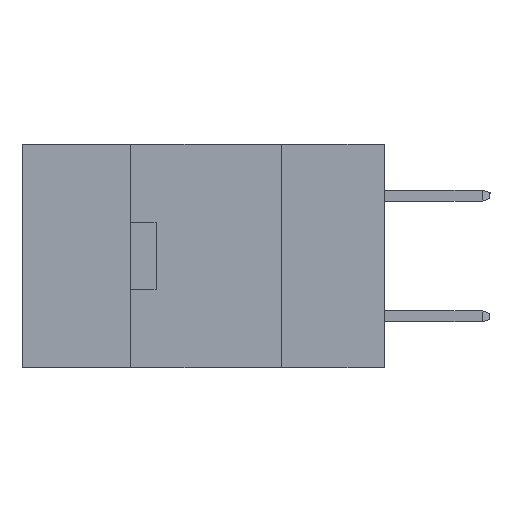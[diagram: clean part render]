
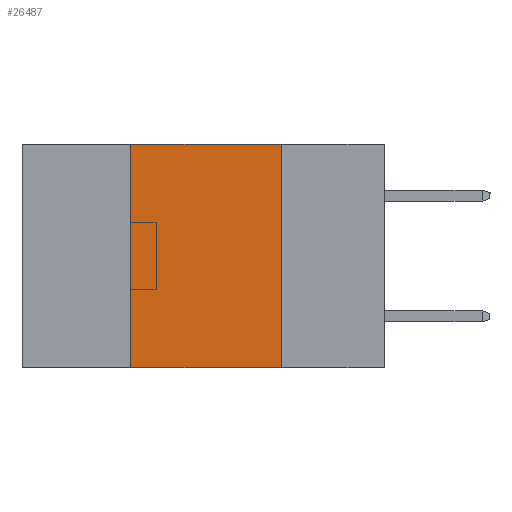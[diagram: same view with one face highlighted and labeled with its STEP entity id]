
A CAD part, left-side view. The second image highlights one B-rep face of the part: STEP entity #26487.
In plain terms, the highlighted planar face has unit normal (-1, 0, 0).
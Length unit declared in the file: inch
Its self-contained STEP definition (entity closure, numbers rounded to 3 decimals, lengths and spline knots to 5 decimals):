
#595 = VECTOR ( 'NONE', #14069, 39.37008 ) ;
#933 = CARTESIAN_POINT ( 'NONE',  ( 0., 0.6, 0. ) ) ;
#2330 = LINE ( 'NONE', #17750, #13727 ) ;
#3131 = DIRECTION ( 'NONE',  ( 0., 0., -1. ) ) ;
#3324 = CARTESIAN_POINT ( 'NONE',  ( 0., 0.42, 0. ) ) ;
#3597 = ORIENTED_EDGE ( 'NONE', *, *, #27818, .F. ) ;
#4238 = AXIS2_PLACEMENT_3D ( 'NONE', #933, #5519, #7417 ) ;
#5519 = DIRECTION ( 'NONE',  ( 1., 0., 0. ) ) ;
#7417 = DIRECTION ( 'NONE',  ( 0., 0., -1. ) ) ;
#8275 = VERTEX_POINT ( 'NONE', #3324 ) ;
#8822 = DIRECTION ( 'NONE',  ( 0., 0., 1. ) ) ;
#9451 = VERTEX_POINT ( 'NONE', #28411 ) ;
#10268 = CARTESIAN_POINT ( 'NONE',  ( 0., 0.17, 0. ) ) ;
#10902 = LINE ( 'NONE', #21964, #14322 ) ;
#11757 = PLANE ( 'NONE',  #4238 ) ;
#12780 = EDGE_CURVE ( 'NONE', #9451, #8275, #2330, .T. ) ;
#13727 = VECTOR ( 'NONE', #8822, 39.37008 ) ;
#14053 = FACE_OUTER_BOUND ( 'NONE', #19999, .T. ) ;
#14069 = DIRECTION ( 'NONE',  ( 0., -1., 0. ) ) ;
#14322 = VECTOR ( 'NONE', #17942, 39.37008 ) ;
#14664 = VERTEX_POINT ( 'NONE', #25762 ) ;
#17750 = CARTESIAN_POINT ( 'NONE',  ( 0., 0.42, -0.37 ) ) ;
#17942 = DIRECTION ( 'NONE',  ( 0., -1., 0. ) ) ;
#18158 = ORIENTED_EDGE ( 'NONE', *, *, #25141, .T. ) ;
#18602 = ORIENTED_EDGE ( 'NONE', *, *, #20578, .F. ) ;
#18658 = CARTESIAN_POINT ( 'NONE',  ( 0., 0.6, 0. ) ) ;
#19999 = EDGE_LOOP ( 'NONE', ( #3597, #18602, #20051, #18158 ) ) ;
#20051 = ORIENTED_EDGE ( 'NONE', *, *, #12780, .F. ) ;
#20578 = EDGE_CURVE ( 'NONE', #8275, #25824, #25427, .T. ) ;
#21964 = CARTESIAN_POINT ( 'NONE',  ( 0., 0.6, -0.37 ) ) ;
#24083 = VECTOR ( 'NONE', #3131, 39.37008 ) ;
#24753 = CARTESIAN_POINT ( 'NONE',  ( 0., 0.17, -0.37 ) ) ;
#25141 = EDGE_CURVE ( 'NONE', #9451, #14664, #10902, .T. ) ;
#25427 = LINE ( 'NONE', #18658, #595 ) ;
#25762 = CARTESIAN_POINT ( 'NONE',  ( 0., 0.17, -0.37 ) ) ;
#25824 = VERTEX_POINT ( 'NONE', #10268 ) ;
#26212 = LINE ( 'NONE', #24753, #24083 ) ;
#26487 = ADVANCED_FACE ( 'NONE', ( #14053 ), #11757, .F. ) ;
#27818 = EDGE_CURVE ( 'NONE', #25824, #14664, #26212, .T. ) ;
#28411 = CARTESIAN_POINT ( 'NONE',  ( 0., 0.42, -0.37 ) ) ;
